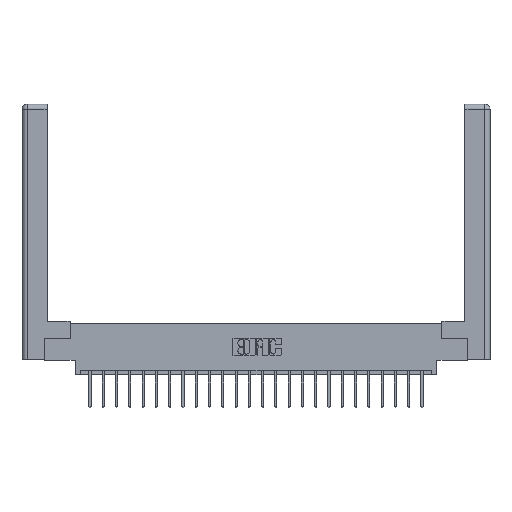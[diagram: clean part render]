
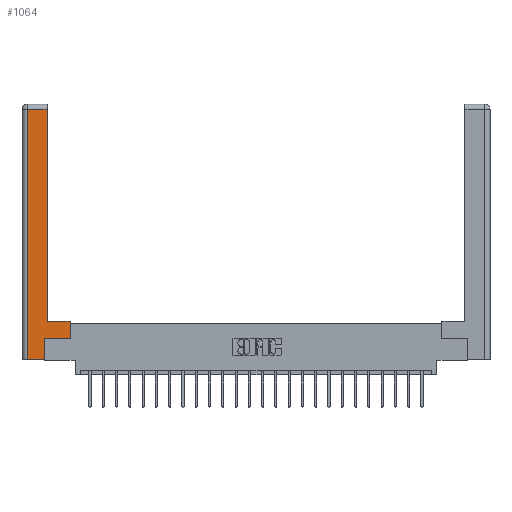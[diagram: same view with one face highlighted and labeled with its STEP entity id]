
A CAD part, top view. The second image highlights one B-rep face of the part: STEP entity #1064.
In plain terms, the highlighted planar face has unit normal (0, 0, 1).
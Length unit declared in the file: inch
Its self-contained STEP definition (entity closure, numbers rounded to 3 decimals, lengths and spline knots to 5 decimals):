
#146 = VERTEX_POINT ( 'NONE', #2821 ) ;
#240 = DIRECTION ( 'NONE',  ( 1., 0., 0. ) ) ;
#492 = CARTESIAN_POINT ( 'NONE',  ( 0.265, 0.245, 0. ) ) ;
#1054 = VECTOR ( 'NONE', #20109, 39.37008 ) ;
#1064 = ADVANCED_FACE ( 'NONE', ( #8382 ), #22942, .F. ) ;
#1195 = ORIENTED_EDGE ( 'NONE', *, *, #19340, .T. ) ;
#1628 = CARTESIAN_POINT ( 'NONE',  ( 0.265, 0., 0. ) ) ;
#1866 = EDGE_LOOP ( 'NONE', ( #4785, #10597, #1195, #9488, #24450, #6946, #14787, #21153 ) ) ;
#2085 = VECTOR ( 'NONE', #4278, 39.37008 ) ;
#2586 = CARTESIAN_POINT ( 'NONE',  ( 0.0615, 2.94, 0. ) ) ;
#2821 = CARTESIAN_POINT ( 'NONE',  ( 0.265, 0., 0. ) ) ;
#3003 = AXIS2_PLACEMENT_3D ( 'NONE', #18842, #24866, #24703 ) ;
#3393 = VERTEX_POINT ( 'NONE', #13338 ) ;
#3490 = VECTOR ( 'NONE', #14190, 39.37008 ) ;
#3849 = DIRECTION ( 'NONE',  ( 0., 1., 0. ) ) ;
#4278 = DIRECTION ( 'NONE',  ( 0., 1., 0. ) ) ;
#4785 = ORIENTED_EDGE ( 'NONE', *, *, #19380, .T. ) ;
#4911 = EDGE_CURVE ( 'NONE', #5817, #23619, #18628, .T. ) ;
#5817 = VERTEX_POINT ( 'NONE', #9780 ) ;
#6051 = CARTESIAN_POINT ( 'NONE',  ( 0.565, 0.45, 0. ) ) ;
#6946 = ORIENTED_EDGE ( 'NONE', *, *, #7314, .T. ) ;
#7314 = EDGE_CURVE ( 'NONE', #11226, #13062, #8288, .T. ) ;
#7349 = CARTESIAN_POINT ( 'NONE',  ( 0.565, 0.245, 0. ) ) ;
#7829 = EDGE_CURVE ( 'NONE', #14490, #146, #24268, .T. ) ;
#8124 = VECTOR ( 'NONE', #17884, 39.37008 ) ;
#8288 = LINE ( 'NONE', #7349, #16686 ) ;
#8382 = FACE_OUTER_BOUND ( 'NONE', #1866, .T. ) ;
#9311 = DIRECTION ( 'NONE',  ( -1., 0., 0. ) ) ;
#9488 = ORIENTED_EDGE ( 'NONE', *, *, #7829, .T. ) ;
#9744 = CARTESIAN_POINT ( 'NONE',  ( 0.565, 0.45, 0. ) ) ;
#9780 = CARTESIAN_POINT ( 'NONE',  ( 0.295, 2.94, 0. ) ) ;
#10597 = ORIENTED_EDGE ( 'NONE', *, *, #4911, .T. ) ;
#11226 = VERTEX_POINT ( 'NONE', #492 ) ;
#11318 = LINE ( 'NONE', #21754, #1054 ) ;
#12508 = LINE ( 'NONE', #17921, #3490 ) ;
#13062 = VERTEX_POINT ( 'NONE', #13563 ) ;
#13121 = VECTOR ( 'NONE', #3849, 39.37008 ) ;
#13139 = DIRECTION ( 'NONE',  ( 1., 0., 0. ) ) ;
#13338 = CARTESIAN_POINT ( 'NONE',  ( 0.295, 0.45, 0. ) ) ;
#13563 = CARTESIAN_POINT ( 'NONE',  ( 0.565, 0.245, 0. ) ) ;
#14190 = DIRECTION ( 'NONE',  ( 0., -1., 0. ) ) ;
#14490 = VERTEX_POINT ( 'NONE', #22929 ) ;
#14787 = ORIENTED_EDGE ( 'NONE', *, *, #19640, .T. ) ;
#15171 = VECTOR ( 'NONE', #240, 39.37008 ) ;
#16686 = VECTOR ( 'NONE', #13139, 39.37008 ) ;
#16705 = CARTESIAN_POINT ( 'NONE',  ( 0.295, 0.45, 0. ) ) ;
#17178 = VERTEX_POINT ( 'NONE', #6051 ) ;
#17434 = LINE ( 'NONE', #19361, #2085 ) ;
#17884 = DIRECTION ( 'NONE',  ( -1., 0., 0. ) ) ;
#17921 = CARTESIAN_POINT ( 'NONE',  ( 0.0615, 0., 0. ) ) ;
#18232 = LINE ( 'NONE', #9744, #13121 ) ;
#18628 = LINE ( 'NONE', #20576, #8124 ) ;
#18681 = LINE ( 'NONE', #16705, #22030 ) ;
#18842 = CARTESIAN_POINT ( 'NONE',  ( 0., 0., 0. ) ) ;
#19340 = EDGE_CURVE ( 'NONE', #23619, #14490, #12508, .T. ) ;
#19361 = CARTESIAN_POINT ( 'NONE',  ( 0.265, 0.245, 0. ) ) ;
#19380 = EDGE_CURVE ( 'NONE', #3393, #5817, #11318, .T. ) ;
#19640 = EDGE_CURVE ( 'NONE', #13062, #17178, #18232, .T. ) ;
#20109 = DIRECTION ( 'NONE',  ( 0., 1., 0. ) ) ;
#20576 = CARTESIAN_POINT ( 'NONE',  ( 0.0615, 2.94, 0. ) ) ;
#21153 = ORIENTED_EDGE ( 'NONE', *, *, #23910, .T. ) ;
#21754 = CARTESIAN_POINT ( 'NONE',  ( 0.295, 3., 0. ) ) ;
#22030 = VECTOR ( 'NONE', #9311, 39.37008 ) ;
#22929 = CARTESIAN_POINT ( 'NONE',  ( 0.0615, 0., 0. ) ) ;
#22942 = PLANE ( 'NONE',  #3003 ) ;
#23619 = VERTEX_POINT ( 'NONE', #2586 ) ;
#23910 = EDGE_CURVE ( 'NONE', #17178, #3393, #18681, .T. ) ;
#24268 = LINE ( 'NONE', #1628, #15171 ) ;
#24450 = ORIENTED_EDGE ( 'NONE', *, *, #24479, .T. ) ;
#24479 = EDGE_CURVE ( 'NONE', #146, #11226, #17434, .T. ) ;
#24703 = DIRECTION ( 'NONE',  ( -1., 0., 0. ) ) ;
#24866 = DIRECTION ( 'NONE',  ( 0., 0., -1. ) ) ;
